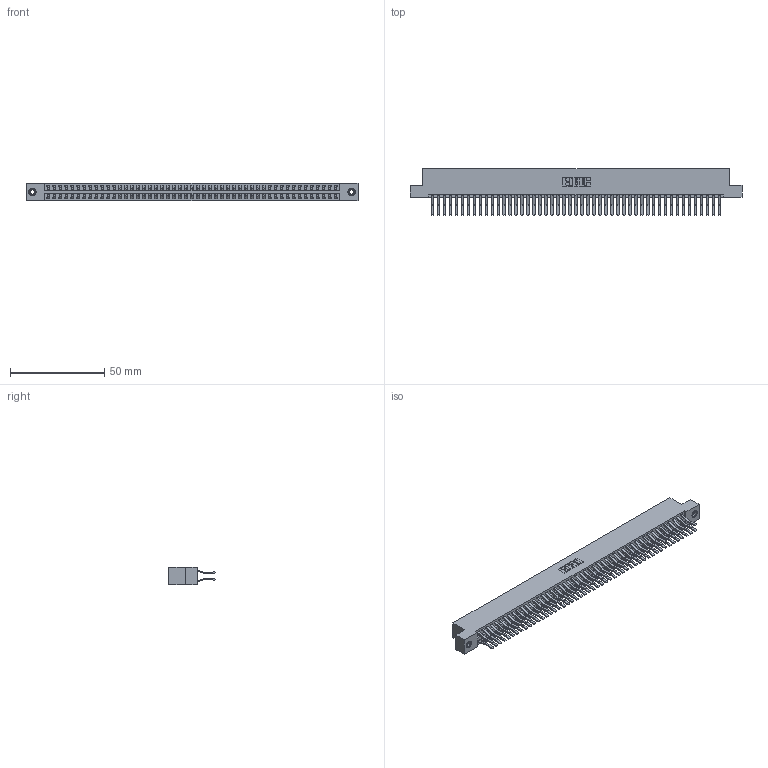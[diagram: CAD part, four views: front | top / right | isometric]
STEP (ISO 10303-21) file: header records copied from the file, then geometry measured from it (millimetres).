
FILE_DESCRIPTION (( 'STEP AP203' ), '1' );
FILE_NAME ('396-098-560-208.STEP', '2018-09-14T06:14:16', ( '' ), ( '' ), 'SwSTEP 2.0', 'SolidWorks 2016', '' );
FILE_SCHEMA (( 'CONFIG_CONTROL_DESIGN' ));
Length unit declared in the file: inch
Products named in the file (4): 346 Part_Flush Mounting Lugs - 0.156 Dia-TI; 345-292-001_560 Tail; 345-250-001_345-250-003-102; 396-098-560-208
Assembly tree (101 placements, depth 2):
  396-098-560-208
    346 Part_Flush Mounting Lugs - 0.156 Dia-TI
    345-292-001_560 Tail  x98
    345-250-001_345-250-003-102  x2
Bounding box: 176.15 x 24.78 x 9.4 mm (x, y, z)
Volume: 17866.9 mm3; surface area: 26403.1 mm2
Topology: 101 solids, 101 shells, 5474 faces, 16243 edges, 10690 vertices
Faces by surface type: plane 3538, cylinder 1920, cone 12, torus 4
Entity records: 32310 total; most frequent: CARTESIAN_POINT 5299, ORIENTED_EDGE 5226, DIRECTION 4751, EDGE_CURVE 2613, VECTOR 2261, LINE 2261, VERTEX_POINT 1736, AXIS2_PLACEMENT_3D 1245
